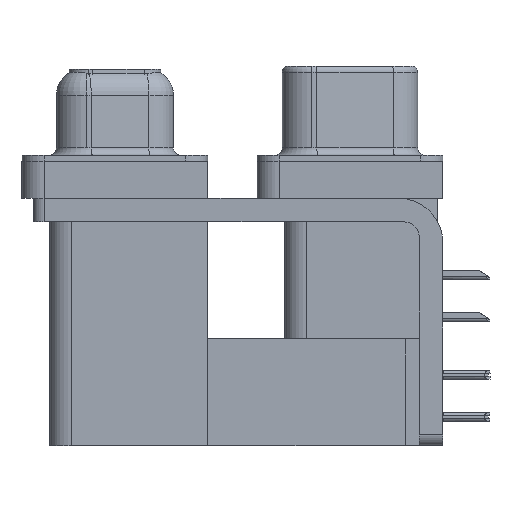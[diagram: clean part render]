
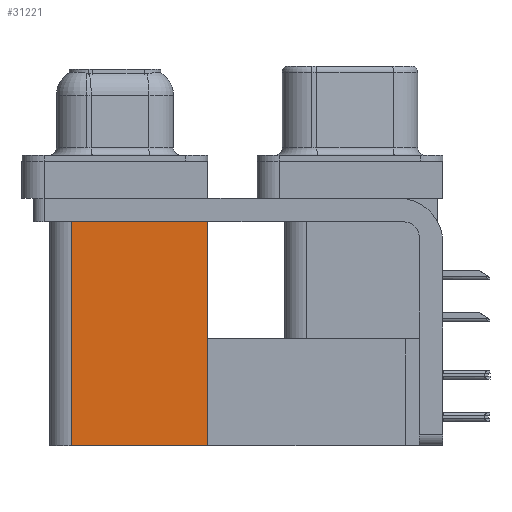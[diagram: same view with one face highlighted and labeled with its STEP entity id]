
A CAD part, left-side view. The second image highlights one B-rep face of the part: STEP entity #31221.
In plain terms, the highlighted planar face has unit normal (-1, 0, 0).
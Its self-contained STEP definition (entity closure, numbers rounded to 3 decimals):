
#699 = DIRECTION ( 'NONE',  ( 0., 0., 1. ) ) ;
#1971 = CARTESIAN_POINT ( 'NONE',  ( 3.765, 9.6, -19.2 ) ) ;
#2346 = VECTOR ( 'NONE', #24520, 1000. ) ;
#2363 = VECTOR ( 'NONE', #699, 1000. ) ;
#2735 = LINE ( 'NONE', #18507, #10430 ) ;
#3374 = VERTEX_POINT ( 'NONE', #38540 ) ;
#4318 = CARTESIAN_POINT ( 'NONE',  ( 3.765, 9.6, -19.2 ) ) ;
#5979 = DIRECTION ( 'NONE',  ( 0., 0., -1. ) ) ;
#7460 = EDGE_CURVE ( 'NONE', #20879, #3374, #27461, .T. ) ;
#7893 = CARTESIAN_POINT ( 'NONE',  ( 3.765, 9.6, -19.2 ) ) ;
#9676 = EDGE_LOOP ( 'NONE', ( #17726, #21816, #28146, #28553 ) ) ;
#10430 = VECTOR ( 'NONE', #21451, 1000. ) ;
#11069 = VERTEX_POINT ( 'NONE', #11911 ) ;
#11911 = CARTESIAN_POINT ( 'NONE',  ( 3.765, 18.8, -19.2 ) ) ;
#13983 = DIRECTION ( 'NONE',  ( 0., 1., 0. ) ) ;
#17726 = ORIENTED_EDGE ( 'NONE', *, *, #7460, .T. ) ;
#17985 = EDGE_CURVE ( 'NONE', #36571, #11069, #23452, .T. ) ;
#18149 = FACE_OUTER_BOUND ( 'NONE', #9676, .T. ) ;
#18507 = CARTESIAN_POINT ( 'NONE',  ( 3.765, 9.6, -19.2 ) ) ;
#20879 = VERTEX_POINT ( 'NONE', #26320 ) ;
#21451 = DIRECTION ( 'NONE',  ( 0., 0., 1. ) ) ;
#21816 = ORIENTED_EDGE ( 'NONE', *, *, #22648, .F. ) ;
#22648 = EDGE_CURVE ( 'NONE', #11069, #3374, #39187, .T. ) ;
#23452 = LINE ( 'NONE', #4318, #29716 ) ;
#23774 = AXIS2_PLACEMENT_3D ( 'NONE', #1971, #27411, #5979 ) ;
#24520 = DIRECTION ( 'NONE',  ( 0., 1., 0. ) ) ;
#24602 = EDGE_CURVE ( 'NONE', #36571, #20879, #2735, .T. ) ;
#26320 = CARTESIAN_POINT ( 'NONE',  ( 3.765, 9.6, -2.5 ) ) ;
#26792 = CARTESIAN_POINT ( 'NONE',  ( 3.765, 18.8, -19.2 ) ) ;
#27411 = DIRECTION ( 'NONE',  ( 1., 0., 0. ) ) ;
#27461 = LINE ( 'NONE', #34595, #2346 ) ;
#28146 = ORIENTED_EDGE ( 'NONE', *, *, #17985, .F. ) ;
#28553 = ORIENTED_EDGE ( 'NONE', *, *, #24602, .T. ) ;
#29716 = VECTOR ( 'NONE', #13983, 1000. ) ;
#31221 = ADVANCED_FACE ( 'NONE', ( #18149 ), #40437, .F. ) ;
#34595 = CARTESIAN_POINT ( 'NONE',  ( 3.765, 9.6, -2.5 ) ) ;
#36571 = VERTEX_POINT ( 'NONE', #7893 ) ;
#38540 = CARTESIAN_POINT ( 'NONE',  ( 3.765, 18.8, -2.5 ) ) ;
#39187 = LINE ( 'NONE', #26792, #2363 ) ;
#40437 = PLANE ( 'NONE',  #23774 ) ;
